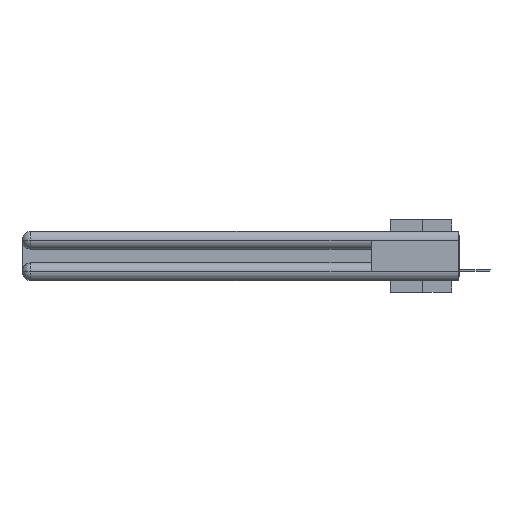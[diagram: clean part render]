
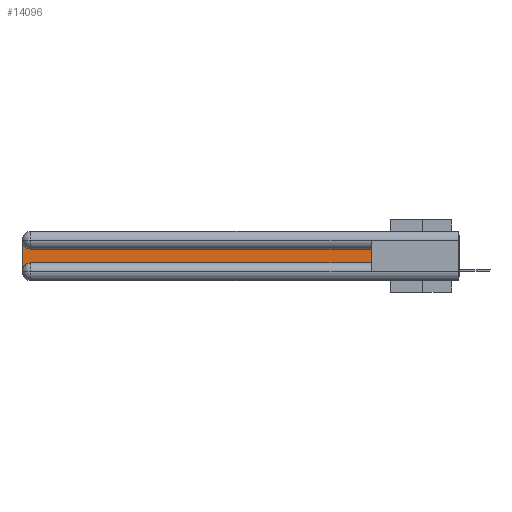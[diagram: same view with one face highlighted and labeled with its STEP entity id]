
A CAD part, left-side view. The second image highlights one B-rep face of the part: STEP entity #14096.
In plain terms, the highlighted planar face has unit normal (-1, 0, 0).
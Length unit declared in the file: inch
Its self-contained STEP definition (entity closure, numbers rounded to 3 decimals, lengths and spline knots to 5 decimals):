
#102 = AXIS2_PLACEMENT_3D ( 'NONE', #21574, #17273, #14834 ) ;
#715 = CARTESIAN_POINT ( 'NONE',  ( 0.075, 2.94, -0.2775 ) ) ;
#1753 = PLANE ( 'NONE',  #102 ) ;
#1938 = CIRCLE ( 'NONE', #17596, 0.06 ) ;
#2095 = DIRECTION ( 'NONE',  ( 0., 0., -1. ) ) ;
#2325 = VERTEX_POINT ( 'NONE', #17386 ) ;
#2576 = CARTESIAN_POINT ( 'NONE',  ( 0.075, 0.6, -0.2175 ) ) ;
#3893 = LINE ( 'NONE', #12928, #5296 ) ;
#4146 = CARTESIAN_POINT ( 'NONE',  ( 0.075, 0.6, -0.2175 ) ) ;
#5296 = VECTOR ( 'NONE', #2095, 39.37008 ) ;
#5363 = ORIENTED_EDGE ( 'NONE', *, *, #8126, .T. ) ;
#5465 = ORIENTED_EDGE ( 'NONE', *, *, #18639, .T. ) ;
#5964 = ORIENTED_EDGE ( 'NONE', *, *, #7247, .T. ) ;
#6121 = ORIENTED_EDGE ( 'NONE', *, *, #15367, .T. ) ;
#6576 = DIRECTION ( 'NONE',  ( 0., -1., 0. ) ) ;
#6795 = DIRECTION ( 'NONE',  ( 0., 0., 1. ) ) ;
#7247 = EDGE_CURVE ( 'NONE', #27559, #19369, #9266, .T. ) ;
#7600 = CARTESIAN_POINT ( 'NONE',  ( 0.075, 2.94, -0.0625 ) ) ;
#8126 = EDGE_CURVE ( 'NONE', #2325, #27559, #26633, .T. ) ;
#8601 = CARTESIAN_POINT ( 'NONE',  ( 0.075, 3., -0.0625 ) ) ;
#9266 = CIRCLE ( 'NONE', #18569, 0.06 ) ;
#9396 = VERTEX_POINT ( 'NONE', #17815 ) ;
#10858 = CARTESIAN_POINT ( 'NONE',  ( 0.075, 0.6, -0.2175 ) ) ;
#11941 = DIRECTION ( 'NONE',  ( 0., 0., -1. ) ) ;
#12006 = EDGE_LOOP ( 'NONE', ( #5363, #5964, #5465, #18467, #6121, #25704 ) ) ;
#12198 = FACE_OUTER_BOUND ( 'NONE', #12006, .T. ) ;
#12928 = CARTESIAN_POINT ( 'NONE',  ( 0.075, 3., -0.2175 ) ) ;
#14096 = ADVANCED_FACE ( 'NONE', ( #12198 ), #1753, .F. ) ;
#14325 = VECTOR ( 'NONE', #6576, 39.37008 ) ;
#14834 = DIRECTION ( 'NONE',  ( 0., 0., -1. ) ) ;
#14885 = EDGE_CURVE ( 'NONE', #19859, #2325, #25533, .T. ) ;
#15367 = EDGE_CURVE ( 'NONE', #9396, #19859, #26234, .T. ) ;
#17273 = DIRECTION ( 'NONE',  ( 1., 0., 0. ) ) ;
#17386 = CARTESIAN_POINT ( 'NONE',  ( 0.075, 0.6, -0.1225 ) ) ;
#17596 = AXIS2_PLACEMENT_3D ( 'NONE', #715, #25399, #11941 ) ;
#17815 = CARTESIAN_POINT ( 'NONE',  ( 0.075, 2.94, -0.2175 ) ) ;
#18467 = ORIENTED_EDGE ( 'NONE', *, *, #25577, .T. ) ;
#18569 = AXIS2_PLACEMENT_3D ( 'NONE', #7600, #25548, #18986 ) ;
#18639 = EDGE_CURVE ( 'NONE', #19369, #27768, #3893, .T. ) ;
#18986 = DIRECTION ( 'NONE',  ( 0., 0., -1. ) ) ;
#19369 = VERTEX_POINT ( 'NONE', #8601 ) ;
#19859 = VERTEX_POINT ( 'NONE', #10858 ) ;
#20651 = VECTOR ( 'NONE', #26894, 39.37008 ) ;
#21191 = CARTESIAN_POINT ( 'NONE',  ( 0.075, 2.94, -0.1225 ) ) ;
#21574 = CARTESIAN_POINT ( 'NONE',  ( 0.075, 3., -0.1225 ) ) ;
#22763 = CARTESIAN_POINT ( 'NONE',  ( 0.075, 0.6, -0.1225 ) ) ;
#25399 = DIRECTION ( 'NONE',  ( 1., 0., 0. ) ) ;
#25533 = LINE ( 'NONE', #2576, #26963 ) ;
#25548 = DIRECTION ( 'NONE',  ( 1., 0., 0. ) ) ;
#25577 = EDGE_CURVE ( 'NONE', #27768, #9396, #1938, .T. ) ;
#25704 = ORIENTED_EDGE ( 'NONE', *, *, #14885, .T. ) ;
#26234 = LINE ( 'NONE', #4146, #14325 ) ;
#26633 = LINE ( 'NONE', #22763, #20651 ) ;
#26894 = DIRECTION ( 'NONE',  ( 0., 1., 0. ) ) ;
#26963 = VECTOR ( 'NONE', #6795, 39.37008 ) ;
#27559 = VERTEX_POINT ( 'NONE', #21191 ) ;
#27768 = VERTEX_POINT ( 'NONE', #28387 ) ;
#28387 = CARTESIAN_POINT ( 'NONE',  ( 0.075, 3., -0.2775 ) ) ;
